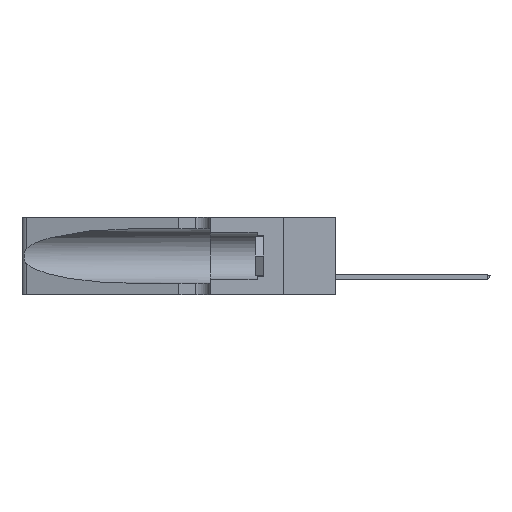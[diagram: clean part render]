
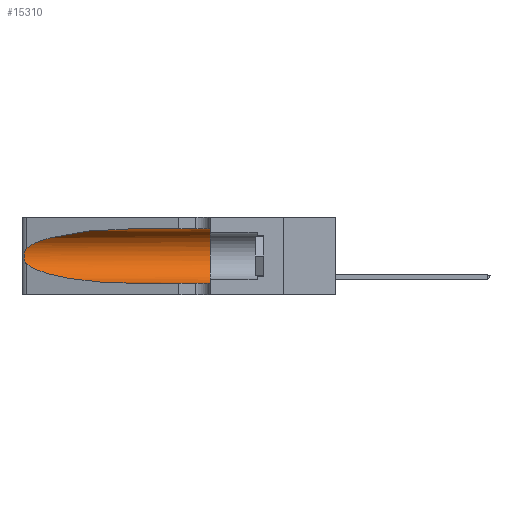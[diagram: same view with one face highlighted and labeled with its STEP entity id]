
A CAD part, left-side view. The second image highlights one B-rep face of the part: STEP entity #15310.
In plain terms, the highlighted cylindrical face has radius 3.308 mm (diameter 6.617 mm), a partial arc.
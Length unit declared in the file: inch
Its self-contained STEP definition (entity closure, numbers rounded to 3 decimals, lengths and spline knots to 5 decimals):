
#742 = CARTESIAN_POINT ( 'NONE',  ( 0.26075, 1.23896, 0.19203 ) ) ;
#869 = CARTESIAN_POINT ( 'NONE',  ( 0.25639, 1.23184, 0.21858 ) ) ;
#1990 = CARTESIAN_POINT ( 'NONE',  ( 0.1305, 0.35, 0.05475 ) ) ;
#2150 = DIRECTION ( 'NONE',  ( 0., -1., 0. ) ) ;
#2371 =( BOUNDED_CURVE ( )  B_SPLINE_CURVE ( 3, ( #16006, #18768, #10771, #16125 ),
 .UNSPECIFIED., .F., .T. ) 
 B_SPLINE_CURVE_WITH_KNOTS ( ( 4, 4 ),
 ( 3.44316, 4.71239 ),
 .UNSPECIFIED. ) 
 CURVE ( )  GEOMETRIC_REPRESENTATION_ITEM ( )  RATIONAL_B_SPLINE_CURVE ( ( 1., 0.87, 0.87, 1. ) ) 
 REPRESENTATION_ITEM ( '' )  );
#2497 = FACE_OUTER_BOUND ( 'NONE', #28675, .T. ) ;
#3210 = VERTEX_POINT ( 'NONE', #11039 ) ;
#3228 = CARTESIAN_POINT ( 'NONE',  ( 0.26017, 1.23833, 0.17102 ) ) ;
#3460 = CARTESIAN_POINT ( 'NONE',  ( 0.25639, 1.23186, 0.15144 ) ) ;
#4139 = CARTESIAN_POINT ( 'NONE',  ( 0.25787, 1.23484, 0.2124 ) ) ;
#4764 = DIRECTION ( 'NONE',  ( 0., 0., -1. ) ) ;
#5153 = VERTEX_POINT ( 'NONE', #1990 ) ;
#5860 = CARTESIAN_POINT ( 'NONE',  ( 0.25555, 1.22994, 0.2215 ) ) ;
#5933 = AXIS2_PLACEMENT_3D ( 'NONE', #28968, #12554, #26463 ) ;
#6091 = CARTESIAN_POINT ( 'NONE',  ( 0.25854, 1.2359, 0.20912 ) ) ;
#6152 = EDGE_CURVE ( 'NONE', #28549, #24317, #2371, .T. ) ;
#6234 = CARTESIAN_POINT ( 'NONE',  ( 0.25487, 1.22718, 0.14631 ) ) ;
#7267 = ORIENTED_EDGE ( 'NONE', *, *, #12802, .F. ) ;
#8155 = CARTESIAN_POINT ( 'NONE',  ( 0.25487, 1.22718, 0.14631 ) ) ;
#8443 = CARTESIAN_POINT ( 'NONE',  ( 0.1305, 1.61858, 0.05475 ) ) ;
#9328 = CARTESIAN_POINT ( 'NONE',  ( 0.1305, 0.35, 0.31525 ) ) ;
#9331 = CYLINDRICAL_SURFACE ( 'NONE', #15885, 0.13025 ) ;
#9659 = CARTESIAN_POINT ( 'NONE',  ( 0.25789, 1.23486, 0.15765 ) ) ;
#10771 = CARTESIAN_POINT ( 'NONE',  ( 0.18966, 0.96281, 0.05475 ) ) ;
#10797 = ORIENTED_EDGE ( 'NONE', *, *, #27320, .F. ) ;
#11039 = CARTESIAN_POINT ( 'NONE',  ( 0.25487, 1.22718, 0.22369 ) ) ;
#11254 = CARTESIAN_POINT ( 'NONE',  ( 0.1305, 0.72297, 0.31525 ) ) ;
#11695 = EDGE_CURVE ( 'NONE', #11857, #3210, #33712, .T. ) ;
#11857 = VERTEX_POINT ( 'NONE', #21281 ) ;
#12554 = DIRECTION ( 'NONE',  ( 0., 1., 0. ) ) ;
#12802 = EDGE_CURVE ( 'NONE', #20294, #5153, #25655, .T. ) ;
#14592 = B_SPLINE_CURVE_WITH_KNOTS ( 'NONE', 3,
 ( #17235, #5860, #869, #4139, #6091, #17101, #742, #19868, #3228, #25170, #9659, #3460, #22640, #6234 ),
 .UNSPECIFIED., .F., .F.,
 ( 4, 2, 2, 2, 2, 2, 4 ),
 ( 0., 0.00027, 0.00053, 0.00107, 0.0016, 0.00187, 0.00214 ),
 .UNSPECIFIED. ) ;
#15310 = ADVANCED_FACE ( 'NONE', ( #2497 ), #9331, .F. ) ;
#15885 = AXIS2_PLACEMENT_3D ( 'NONE', #24315, #2150, #4764 ) ;
#16006 = CARTESIAN_POINT ( 'NONE',  ( 0.25487, 1.22718, 0.14631 ) ) ;
#16125 = CARTESIAN_POINT ( 'NONE',  ( 0.1305, 0.72297, 0.05475 ) ) ;
#17101 = CARTESIAN_POINT ( 'NONE',  ( 0.26018, 1.23835, 0.19895 ) ) ;
#17235 = CARTESIAN_POINT ( 'NONE',  ( 0.25487, 1.22718, 0.22369 ) ) ;
#17890 = VECTOR ( 'NONE', #27485, 39.37008 ) ;
#17991 = LINE ( 'NONE', #30764, #19643 ) ;
#18768 = CARTESIAN_POINT ( 'NONE',  ( 0.2373, 1.15595, 0.08982 ) ) ;
#19376 = ORIENTED_EDGE ( 'NONE', *, *, #11695, .T. ) ;
#19643 = VECTOR ( 'NONE', #19969, 39.37008 ) ;
#19868 = CARTESIAN_POINT ( 'NONE',  ( 0.26075, 1.23896, 0.178 ) ) ;
#19969 = DIRECTION ( 'NONE',  ( 0., -1., 0. ) ) ;
#19992 = CARTESIAN_POINT ( 'NONE',  ( 0.2373, 1.15595, 0.28018 ) ) ;
#20294 = VERTEX_POINT ( 'NONE', #9328 ) ;
#21281 = CARTESIAN_POINT ( 'NONE',  ( 0.1305, 0.72297, 0.31525 ) ) ;
#21657 = EDGE_CURVE ( 'NONE', #3210, #28549, #14592, .T. ) ;
#22104 = ORIENTED_EDGE ( 'NONE', *, *, #6152, .T. ) ;
#22640 = CARTESIAN_POINT ( 'NONE',  ( 0.25555, 1.22993, 0.14849 ) ) ;
#24315 = CARTESIAN_POINT ( 'NONE',  ( 0.1305, 1.61858, 0.185 ) ) ;
#24317 = VERTEX_POINT ( 'NONE', #34856 ) ;
#25155 = CARTESIAN_POINT ( 'NONE',  ( 0.25487, 1.22718, 0.22369 ) ) ;
#25170 = CARTESIAN_POINT ( 'NONE',  ( 0.25856, 1.23593, 0.16098 ) ) ;
#25441 = ORIENTED_EDGE ( 'NONE', *, *, #29138, .T. ) ;
#25655 = CIRCLE ( 'NONE', #5933, 0.13025 ) ;
#26305 = ORIENTED_EDGE ( 'NONE', *, *, #21657, .T. ) ;
#26463 = DIRECTION ( 'NONE',  ( 0., 0., 1. ) ) ;
#27320 = EDGE_CURVE ( 'NONE', #11857, #20294, #17991, .T. ) ;
#27485 = DIRECTION ( 'NONE',  ( 0., -1., 0. ) ) ;
#28549 = VERTEX_POINT ( 'NONE', #8155 ) ;
#28675 = EDGE_LOOP ( 'NONE', ( #19376, #26305, #22104, #25441, #7267, #10797 ) ) ;
#28968 = CARTESIAN_POINT ( 'NONE',  ( 0.1305, 0.35, 0.185 ) ) ;
#29083 = LINE ( 'NONE', #8443, #17890 ) ;
#29138 = EDGE_CURVE ( 'NONE', #24317, #5153, #29083, .T. ) ;
#30764 = CARTESIAN_POINT ( 'NONE',  ( 0.1305, 1.61858, 0.31525 ) ) ;
#30906 = CARTESIAN_POINT ( 'NONE',  ( 0.18966, 0.96281, 0.31525 ) ) ;
#33712 =( BOUNDED_CURVE ( )  B_SPLINE_CURVE ( 3, ( #11254, #30906, #19992, #25155 ),
 .UNSPECIFIED., .F., .T. ) 
 B_SPLINE_CURVE_WITH_KNOTS ( ( 4, 4 ),
 ( 1.5708, 2.84003 ),
 .UNSPECIFIED. ) 
 CURVE ( )  GEOMETRIC_REPRESENTATION_ITEM ( )  RATIONAL_B_SPLINE_CURVE ( ( 1., 0.87, 0.87, 1. ) ) 
 REPRESENTATION_ITEM ( '' )  );
#34856 = CARTESIAN_POINT ( 'NONE',  ( 0.1305, 0.72297, 0.05475 ) ) ;
